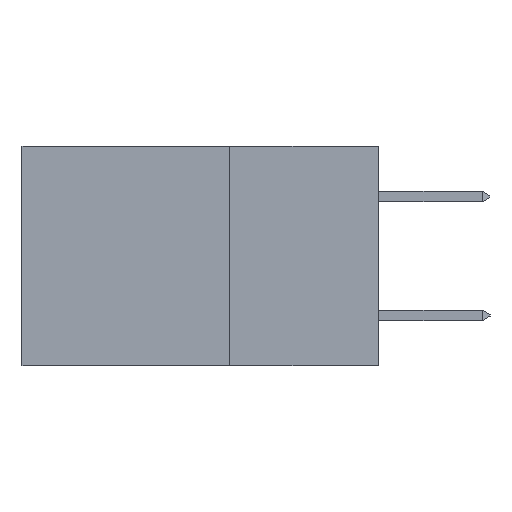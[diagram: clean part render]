
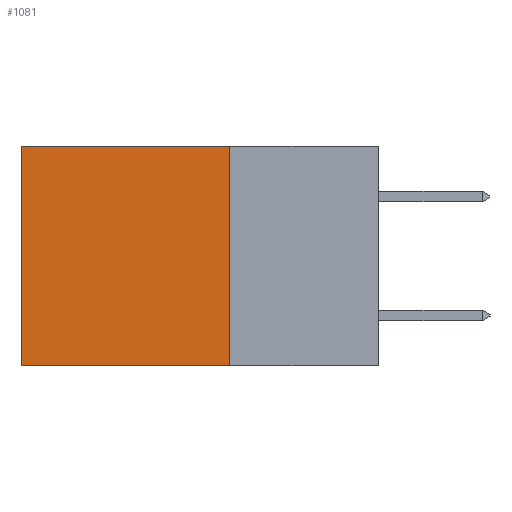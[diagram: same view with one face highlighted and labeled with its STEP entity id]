
A CAD part, left-side view. The second image highlights one B-rep face of the part: STEP entity #1081.
In plain terms, the highlighted planar face has unit normal (-1, 0, 0).
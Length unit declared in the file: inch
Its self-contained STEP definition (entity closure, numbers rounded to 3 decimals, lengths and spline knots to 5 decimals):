
#71 = DIRECTION ( 'NONE',  ( 0., 0., -1. ) ) ;
#290 = VECTOR ( 'NONE', #7896, 39.37008 ) ;
#446 = CARTESIAN_POINT ( 'NONE',  ( 0.2615, 0.25, -0.37 ) ) ;
#471 = CARTESIAN_POINT ( 'NONE',  ( 0.2615, 0.6, -0.37 ) ) ;
#488 = DIRECTION ( 'NONE',  ( 0., 0., -1. ) ) ;
#557 = FACE_OUTER_BOUND ( 'NONE', #9020, .T. ) ;
#770 = ORIENTED_EDGE ( 'NONE', *, *, #2162, .F. ) ;
#1081 = ADVANCED_FACE ( 'NONE', ( #557 ), #2718, .F. ) ;
#1254 = VERTEX_POINT ( 'NONE', #7275 ) ;
#1399 = ORIENTED_EDGE ( 'NONE', *, *, #1577, .T. ) ;
#1577 = EDGE_CURVE ( 'NONE', #7597, #3995, #2329, .T. ) ;
#1754 = VECTOR ( 'NONE', #71, 39.37008 ) ;
#1772 = DIRECTION ( 'NONE',  ( 0., 0., -1. ) ) ;
#2162 = EDGE_CURVE ( 'NONE', #7597, #1254, #9405, .T. ) ;
#2329 = LINE ( 'NONE', #4997, #290 ) ;
#2515 = LINE ( 'NONE', #471, #4298 ) ;
#2542 = CARTESIAN_POINT ( 'NONE',  ( 0.2615, 0.25, -0.37 ) ) ;
#2718 = PLANE ( 'NONE',  #5425 ) ;
#3732 = CARTESIAN_POINT ( 'NONE',  ( 0.2615, 0.6, 0. ) ) ;
#3828 = DIRECTION ( 'NONE',  ( 0., 1., 0. ) ) ;
#3893 = CARTESIAN_POINT ( 'NONE',  ( 0.2615, 0.25, -0.37 ) ) ;
#3972 = CARTESIAN_POINT ( 'NONE',  ( 0.2615, 0.25, 0. ) ) ;
#3995 = VERTEX_POINT ( 'NONE', #3732 ) ;
#4169 = VECTOR ( 'NONE', #3828, 39.37008 ) ;
#4298 = VECTOR ( 'NONE', #488, 39.37008 ) ;
#4958 = EDGE_CURVE ( 'NONE', #3995, #6466, #2515, .T. ) ;
#4997 = CARTESIAN_POINT ( 'NONE',  ( 0.2615, 0.25, 0. ) ) ;
#5425 = AXIS2_PLACEMENT_3D ( 'NONE', #2542, #6364, #1772 ) ;
#5588 = EDGE_CURVE ( 'NONE', #1254, #6466, #6158, .T. ) ;
#5763 = CARTESIAN_POINT ( 'NONE',  ( 0.2615, 0.6, -0.37 ) ) ;
#6158 = LINE ( 'NONE', #3893, #4169 ) ;
#6364 = DIRECTION ( 'NONE',  ( 1., 0., 0. ) ) ;
#6442 = ORIENTED_EDGE ( 'NONE', *, *, #5588, .F. ) ;
#6466 = VERTEX_POINT ( 'NONE', #5763 ) ;
#7221 = ORIENTED_EDGE ( 'NONE', *, *, #4958, .T. ) ;
#7275 = CARTESIAN_POINT ( 'NONE',  ( 0.2615, 0.25, -0.37 ) ) ;
#7597 = VERTEX_POINT ( 'NONE', #3972 ) ;
#7896 = DIRECTION ( 'NONE',  ( 0., 1., 0. ) ) ;
#9020 = EDGE_LOOP ( 'NONE', ( #7221, #6442, #770, #1399 ) ) ;
#9405 = LINE ( 'NONE', #446, #1754 ) ;
